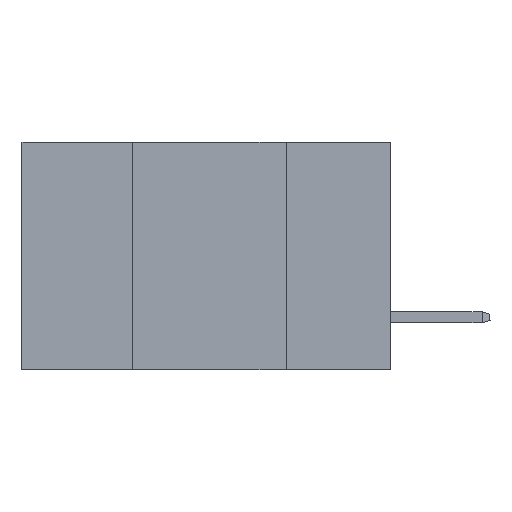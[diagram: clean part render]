
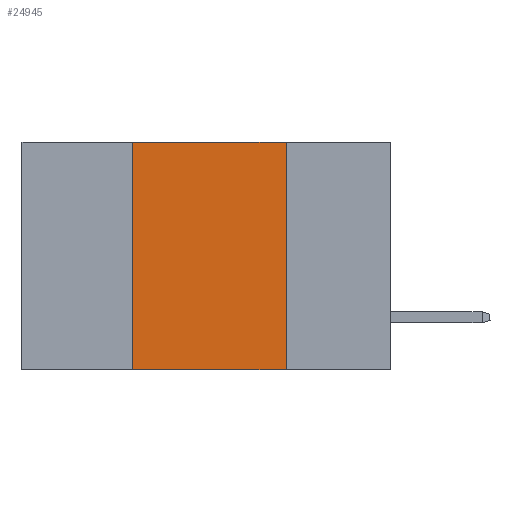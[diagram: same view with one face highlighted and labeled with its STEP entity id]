
A CAD part, left-side view. The second image highlights one B-rep face of the part: STEP entity #24945.
In plain terms, the highlighted planar face has unit normal (-1, 0, 0).
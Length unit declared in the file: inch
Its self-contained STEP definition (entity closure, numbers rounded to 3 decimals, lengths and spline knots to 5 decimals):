
#1027 = LINE ( 'NONE', #36149, #19745 ) ;
#5756 = LINE ( 'NONE', #43112, #21252 ) ;
#9339 = LINE ( 'NONE', #48085, #36667 ) ;
#11412 = CARTESIAN_POINT ( 'NONE',  ( 0., 0.42, -0.37 ) ) ;
#11793 = PLANE ( 'NONE',  #12411 ) ;
#12390 = DIRECTION ( 'NONE',  ( 0., 0., -1. ) ) ;
#12411 = AXIS2_PLACEMENT_3D ( 'NONE', #32085, #36086, #20250 ) ;
#13249 = FACE_OUTER_BOUND ( 'NONE', #32690, .T. ) ;
#15651 = CARTESIAN_POINT ( 'NONE',  ( 0., 0.17, -0.37 ) ) ;
#15741 = DIRECTION ( 'NONE',  ( 0., -1., 0. ) ) ;
#16316 = CARTESIAN_POINT ( 'NONE',  ( 0., 0.42, 0. ) ) ;
#16478 = DIRECTION ( 'NONE',  ( 0., -1., 0. ) ) ;
#18663 = ORIENTED_EDGE ( 'NONE', *, *, #48188, .F. ) ;
#19745 = VECTOR ( 'NONE', #24637, 39.37008 ) ;
#19895 = ORIENTED_EDGE ( 'NONE', *, *, #21893, .F. ) ;
#20250 = DIRECTION ( 'NONE',  ( 0., 0., -1. ) ) ;
#21252 = VECTOR ( 'NONE', #15741, 39.37008 ) ;
#21893 = EDGE_CURVE ( 'NONE', #38338, #50525, #9339, .T. ) ;
#24637 = DIRECTION ( 'NONE',  ( 0., 0., 1. ) ) ;
#24945 = ADVANCED_FACE ( 'NONE', ( #13249 ), #11793, .F. ) ;
#25796 = VERTEX_POINT ( 'NONE', #16316 ) ;
#26584 = VECTOR ( 'NONE', #16478, 39.37008 ) ;
#31027 = EDGE_CURVE ( 'NONE', #25796, #38338, #40240, .T. ) ;
#32085 = CARTESIAN_POINT ( 'NONE',  ( 0., 0.6, 0. ) ) ;
#32690 = EDGE_LOOP ( 'NONE', ( #19895, #39568, #18663, #51359 ) ) ;
#33181 = VERTEX_POINT ( 'NONE', #11412 ) ;
#35560 = CARTESIAN_POINT ( 'NONE',  ( 0., 0.6, 0. ) ) ;
#36086 = DIRECTION ( 'NONE',  ( 1., 0., 0. ) ) ;
#36149 = CARTESIAN_POINT ( 'NONE',  ( 0., 0.42, 0. ) ) ;
#36667 = VECTOR ( 'NONE', #12390, 39.37008 ) ;
#38338 = VERTEX_POINT ( 'NONE', #48373 ) ;
#39568 = ORIENTED_EDGE ( 'NONE', *, *, #31027, .F. ) ;
#40240 = LINE ( 'NONE', #35560, #26584 ) ;
#43089 = EDGE_CURVE ( 'NONE', #33181, #50525, #5756, .T. ) ;
#43112 = CARTESIAN_POINT ( 'NONE',  ( 0., 0.6, -0.37 ) ) ;
#48085 = CARTESIAN_POINT ( 'NONE',  ( 0., 0.17, 0. ) ) ;
#48188 = EDGE_CURVE ( 'NONE', #33181, #25796, #1027, .T. ) ;
#48373 = CARTESIAN_POINT ( 'NONE',  ( 0., 0.17, 0. ) ) ;
#50525 = VERTEX_POINT ( 'NONE', #15651 ) ;
#51359 = ORIENTED_EDGE ( 'NONE', *, *, #43089, .T. ) ;
